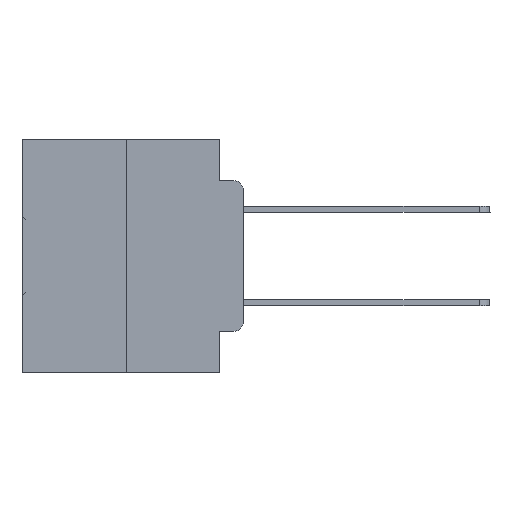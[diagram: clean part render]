
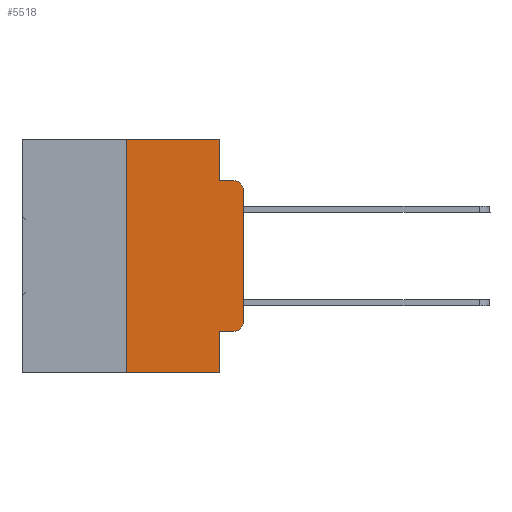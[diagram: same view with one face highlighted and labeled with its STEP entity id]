
A CAD part, left-side view. The second image highlights one B-rep face of the part: STEP entity #5518.
In plain terms, the highlighted planar face has unit normal (-1, 0, 0).
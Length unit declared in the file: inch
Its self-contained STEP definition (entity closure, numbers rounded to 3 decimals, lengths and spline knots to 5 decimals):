
#55 = VERTEX_POINT ( 'NONE', #20552 ) ;
#346 = ORIENTED_EDGE ( 'NONE', *, *, #31162, .T. ) ;
#653 = CARTESIAN_POINT ( 'NONE',  ( 0., 0.473, 0. ) ) ;
#1128 = DIRECTION ( 'NONE',  ( 0., 0., -1. ) ) ;
#1905 = VECTOR ( 'NONE', #22487, 39.37008 ) ;
#3201 = DIRECTION ( 'NONE',  ( 0., 0., -1. ) ) ;
#3725 = CARTESIAN_POINT ( 'NONE',  ( 0., 0.02, -0.1085 ) ) ;
#4260 = AXIS2_PLACEMENT_3D ( 'NONE', #26854, #23926, #18428 ) ;
#4826 = DIRECTION ( 'NONE',  ( 0., -1., 0. ) ) ;
#5285 = VECTOR ( 'NONE', #12967, 39.37008 ) ;
#5518 = ADVANCED_FACE ( 'NONE', ( #24106 ), #15316, .F. ) ;
#6519 = CARTESIAN_POINT ( 'NONE',  ( 0., 0.051, -0.5 ) ) ;
#6522 = VERTEX_POINT ( 'NONE', #9541 ) ;
#7145 = VECTOR ( 'NONE', #4826, 39.37008 ) ;
#7949 = EDGE_CURVE ( 'NONE', #33913, #9254, #17137, .T. ) ;
#8193 = VECTOR ( 'NONE', #27413, 39.37008 ) ;
#8427 = AXIS2_PLACEMENT_3D ( 'NONE', #28805, #14521, #1128 ) ;
#9211 = VERTEX_POINT ( 'NONE', #14577 ) ;
#9254 = VERTEX_POINT ( 'NONE', #6519 ) ;
#9285 = EDGE_CURVE ( 'NONE', #17310, #6522, #25759, .T. ) ;
#9541 = CARTESIAN_POINT ( 'NONE',  ( 0., 0.051, 0. ) ) ;
#10687 = ORIENTED_EDGE ( 'NONE', *, *, #24638, .F. ) ;
#11672 = CARTESIAN_POINT ( 'NONE',  ( 0., 0.25, 0. ) ) ;
#12193 = CARTESIAN_POINT ( 'NONE',  ( 0., 0.051, 0. ) ) ;
#12967 = DIRECTION ( 'NONE',  ( 0., 0., -1. ) ) ;
#13116 = CIRCLE ( 'NONE', #8427, 0.02 ) ;
#13860 = ORIENTED_EDGE ( 'NONE', *, *, #20041, .F. ) ;
#14521 = DIRECTION ( 'NONE',  ( -1., 0., 0. ) ) ;
#14577 = CARTESIAN_POINT ( 'NONE',  ( 0., 0.02, -0.0885 ) ) ;
#14646 = EDGE_CURVE ( 'NONE', #16342, #55, #23002, .T. ) ;
#15316 = PLANE ( 'NONE',  #4260 ) ;
#15393 = EDGE_CURVE ( 'NONE', #20319, #9254, #25086, .T. ) ;
#15681 = VECTOR ( 'NONE', #3201, 39.37008 ) ;
#16342 = VERTEX_POINT ( 'NONE', #35876 ) ;
#16900 = EDGE_CURVE ( 'NONE', #26444, #16342, #13116, .T. ) ;
#17137 = LINE ( 'NONE', #12193, #15681 ) ;
#17310 = VERTEX_POINT ( 'NONE', #28936 ) ;
#17698 = EDGE_CURVE ( 'NONE', #33913, #26444, #24703, .T. ) ;
#17705 = ORIENTED_EDGE ( 'NONE', *, *, #14646, .T. ) ;
#17851 = DIRECTION ( 'NONE',  ( -1., 0., 0. ) ) ;
#18428 = DIRECTION ( 'NONE',  ( 0., 0., -1. ) ) ;
#18464 = LINE ( 'NONE', #27253, #5285 ) ;
#19401 = EDGE_CURVE ( 'NONE', #21705, #9211, #29606, .T. ) ;
#19404 = CARTESIAN_POINT ( 'NONE',  ( 0., 0.051, -0.4115 ) ) ;
#19541 = DIRECTION ( 'NONE',  ( 0., 0., 1. ) ) ;
#19992 = VECTOR ( 'NONE', #35709, 39.37008 ) ;
#20014 = ORIENTED_EDGE ( 'NONE', *, *, #15393, .T. ) ;
#20041 = EDGE_CURVE ( 'NONE', #6522, #21705, #18464, .T. ) ;
#20085 = CARTESIAN_POINT ( 'NONE',  ( 0., 0., 0. ) ) ;
#20319 = VERTEX_POINT ( 'NONE', #20962 ) ;
#20552 = CARTESIAN_POINT ( 'NONE',  ( 0., 0., -0.1085 ) ) ;
#20962 = CARTESIAN_POINT ( 'NONE',  ( 0., 0.25, -0.5 ) ) ;
#21529 = ORIENTED_EDGE ( 'NONE', *, *, #7949, .F. ) ;
#21631 = ORIENTED_EDGE ( 'NONE', *, *, #19401, .F. ) ;
#21705 = VERTEX_POINT ( 'NONE', #24277 ) ;
#22487 = DIRECTION ( 'NONE',  ( 0., 0., 1. ) ) ;
#23002 = LINE ( 'NONE', #20085, #34548 ) ;
#23060 = ORIENTED_EDGE ( 'NONE', *, *, #16900, .T. ) ;
#23215 = LINE ( 'NONE', #11672, #1905 ) ;
#23926 = DIRECTION ( 'NONE',  ( 1., 0., 0. ) ) ;
#24106 = FACE_OUTER_BOUND ( 'NONE', #29846, .T. ) ;
#24277 = CARTESIAN_POINT ( 'NONE',  ( 0., 0.051, -0.0885 ) ) ;
#24638 = EDGE_CURVE ( 'NONE', #20319, #17310, #23215, .T. ) ;
#24703 = LINE ( 'NONE', #19404, #35950 ) ;
#25086 = LINE ( 'NONE', #33146, #19992 ) ;
#25196 = CARTESIAN_POINT ( 'NONE',  ( 0., 0.02, -0.4115 ) ) ;
#25556 = DIRECTION ( 'NONE',  ( 0., 0., -1. ) ) ;
#25759 = LINE ( 'NONE', #653, #7145 ) ;
#26444 = VERTEX_POINT ( 'NONE', #25196 ) ;
#26638 = CIRCLE ( 'NONE', #31974, 0.02 ) ;
#26854 = CARTESIAN_POINT ( 'NONE',  ( 0., 0.473, 0. ) ) ;
#27253 = CARTESIAN_POINT ( 'NONE',  ( 0., 0.051, 0. ) ) ;
#27413 = DIRECTION ( 'NONE',  ( 0., -1., 0. ) ) ;
#28805 = CARTESIAN_POINT ( 'NONE',  ( 0., 0.02, -0.3915 ) ) ;
#28936 = CARTESIAN_POINT ( 'NONE',  ( 0., 0.25, 0. ) ) ;
#29606 = LINE ( 'NONE', #35301, #8193 ) ;
#29846 = EDGE_LOOP ( 'NONE', ( #17705, #346, #21631, #13860, #29881, #10687, #20014, #21529, #29899, #23060 ) ) ;
#29881 = ORIENTED_EDGE ( 'NONE', *, *, #9285, .F. ) ;
#29899 = ORIENTED_EDGE ( 'NONE', *, *, #17698, .T. ) ;
#30740 = DIRECTION ( 'NONE',  ( 0., -1., 0. ) ) ;
#31162 = EDGE_CURVE ( 'NONE', #55, #9211, #26638, .T. ) ;
#31974 = AXIS2_PLACEMENT_3D ( 'NONE', #3725, #17851, #25556 ) ;
#33146 = CARTESIAN_POINT ( 'NONE',  ( 0., 0.473, -0.5 ) ) ;
#33913 = VERTEX_POINT ( 'NONE', #35901 ) ;
#34548 = VECTOR ( 'NONE', #19541, 39.37008 ) ;
#35301 = CARTESIAN_POINT ( 'NONE',  ( 0., 0.051, -0.0885 ) ) ;
#35709 = DIRECTION ( 'NONE',  ( 0., -1., 0. ) ) ;
#35876 = CARTESIAN_POINT ( 'NONE',  ( 0., 0., -0.3915 ) ) ;
#35901 = CARTESIAN_POINT ( 'NONE',  ( 0., 0.051, -0.4115 ) ) ;
#35950 = VECTOR ( 'NONE', #30740, 39.37008 ) ;
